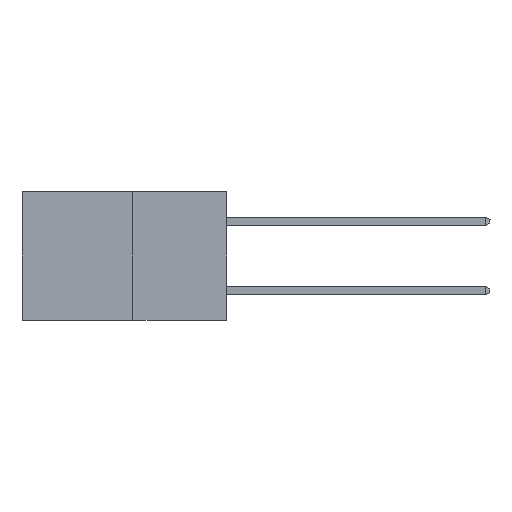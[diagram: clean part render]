
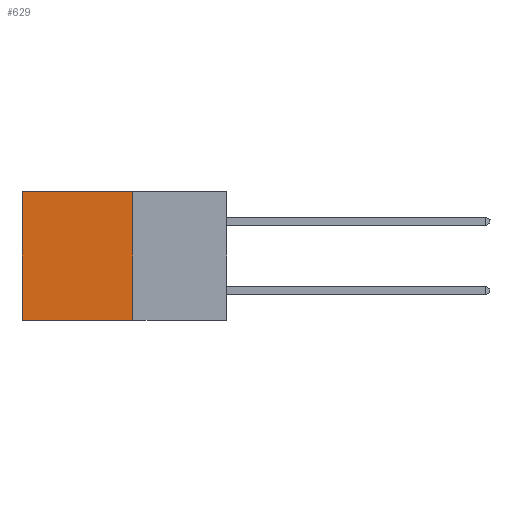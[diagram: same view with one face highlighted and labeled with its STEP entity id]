
A CAD part, left-side view. The second image highlights one B-rep face of the part: STEP entity #629.
In plain terms, the highlighted planar face has unit normal (-1, 0, 0).
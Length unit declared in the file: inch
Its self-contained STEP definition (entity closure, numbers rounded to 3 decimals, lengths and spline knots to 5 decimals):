
#221 = CARTESIAN_POINT ( 'NONE',  ( 0.277, 0.59, -0.37 ) ) ;
#286 = VECTOR ( 'NONE', #540, 39.37008 ) ;
#299 = PLANE ( 'NONE',  #12078 ) ;
#540 = DIRECTION ( 'NONE',  ( 0., 0., -1. ) ) ;
#629 = ADVANCED_FACE ( 'NONE', ( #11164 ), #299, .F. ) ;
#711 = CARTESIAN_POINT ( 'NONE',  ( 0.277, 0.27, -0.37 ) ) ;
#845 = ORIENTED_EDGE ( 'NONE', *, *, #7031, .F. ) ;
#993 = VECTOR ( 'NONE', #5460, 39.37008 ) ;
#1070 = VECTOR ( 'NONE', #5000, 39.37008 ) ;
#1171 = ORIENTED_EDGE ( 'NONE', *, *, #4653, .F. ) ;
#1933 = ORIENTED_EDGE ( 'NONE', *, *, #3285, .T. ) ;
#2638 = VERTEX_POINT ( 'NONE', #3890 ) ;
#3285 = EDGE_CURVE ( 'NONE', #2638, #4218, #10606, .T. ) ;
#3722 = LINE ( 'NONE', #5938, #1070 ) ;
#3890 = CARTESIAN_POINT ( 'NONE',  ( 0.277, 0.59, 0. ) ) ;
#4218 = VERTEX_POINT ( 'NONE', #7733 ) ;
#4269 = VERTEX_POINT ( 'NONE', #11368 ) ;
#4653 = EDGE_CURVE ( 'NONE', #4269, #8894, #10417, .T. ) ;
#5000 = DIRECTION ( 'NONE',  ( 0., 1., 0. ) ) ;
#5421 = VECTOR ( 'NONE', #10560, 39.37008 ) ;
#5458 = CARTESIAN_POINT ( 'NONE',  ( 0.277, 0.27, -0.37 ) ) ;
#5460 = DIRECTION ( 'NONE',  ( 0., 1., 0. ) ) ;
#5938 = CARTESIAN_POINT ( 'NONE',  ( 0.277, 0.27, 0. ) ) ;
#6877 = LINE ( 'NONE', #5458, #993 ) ;
#7031 = EDGE_CURVE ( 'NONE', #8894, #4218, #6877, .T. ) ;
#7064 = DIRECTION ( 'NONE',  ( 0., 0., -1. ) ) ;
#7348 = DIRECTION ( 'NONE',  ( 1., 0., 0. ) ) ;
#7480 = EDGE_LOOP ( 'NONE', ( #1933, #845, #1171, #9893 ) ) ;
#7733 = CARTESIAN_POINT ( 'NONE',  ( 0.277, 0.59, -0.37 ) ) ;
#8894 = VERTEX_POINT ( 'NONE', #11389 ) ;
#9495 = CARTESIAN_POINT ( 'NONE',  ( 0.277, 0.27, -0.37 ) ) ;
#9893 = ORIENTED_EDGE ( 'NONE', *, *, #11140, .T. ) ;
#10417 = LINE ( 'NONE', #711, #286 ) ;
#10560 = DIRECTION ( 'NONE',  ( 0., 0., -1. ) ) ;
#10606 = LINE ( 'NONE', #221, #5421 ) ;
#11140 = EDGE_CURVE ( 'NONE', #4269, #2638, #3722, .T. ) ;
#11164 = FACE_OUTER_BOUND ( 'NONE', #7480, .T. ) ;
#11368 = CARTESIAN_POINT ( 'NONE',  ( 0.277, 0.27, 0. ) ) ;
#11389 = CARTESIAN_POINT ( 'NONE',  ( 0.277, 0.27, -0.37 ) ) ;
#12078 = AXIS2_PLACEMENT_3D ( 'NONE', #9495, #7348, #7064 ) ;
